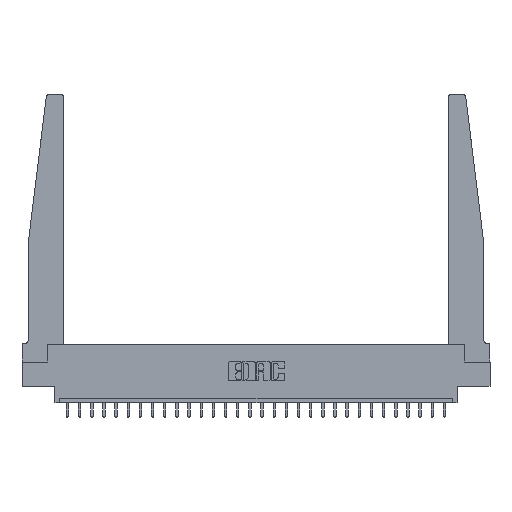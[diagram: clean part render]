
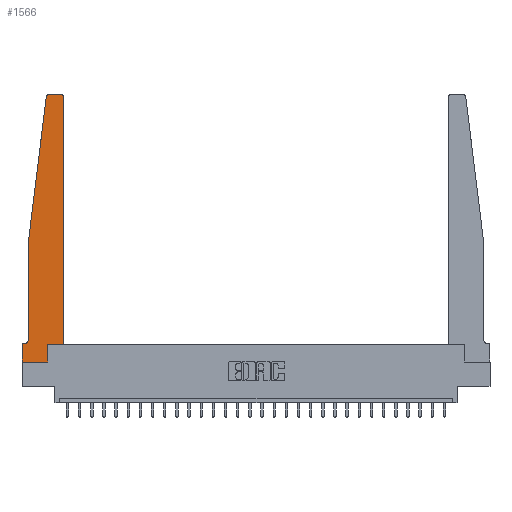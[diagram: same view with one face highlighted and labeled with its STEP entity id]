
A CAD part, top view. The second image highlights one B-rep face of the part: STEP entity #1566.
In plain terms, the highlighted planar face has unit normal (0, 0, 1).
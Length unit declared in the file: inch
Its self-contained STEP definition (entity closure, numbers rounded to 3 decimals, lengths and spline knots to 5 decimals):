
#101 = DIRECTION ( 'NONE',  ( 1., 0., 0. ) ) ;
#103 = VECTOR ( 'NONE', #4401, 39.37008 ) ;
#398 = DIRECTION ( 'NONE',  ( 1., 0., 0. ) ) ;
#920 = VERTEX_POINT ( 'NONE', #13990 ) ;
#1068 = VERTEX_POINT ( 'NONE', #12754 ) ;
#1566 = ADVANCED_FACE ( 'NONE', ( #23547 ), #2660, .T. ) ;
#1679 = DIRECTION ( 'NONE',  ( 0., 0., 1. ) ) ;
#1806 = CIRCLE ( 'NONE', #14305, 0.05 ) ;
#2044 = VECTOR ( 'NONE', #18369, 39.37008 ) ;
#2407 = ORIENTED_EDGE ( 'NONE', *, *, #11332, .T. ) ;
#2491 = VECTOR ( 'NONE', #23407, 39.37008 ) ;
#2496 = VERTEX_POINT ( 'NONE', #19792 ) ;
#2614 = EDGE_CURVE ( 'NONE', #12104, #22840, #1806, .T. ) ;
#2660 = PLANE ( 'NONE',  #24879 ) ;
#2758 = EDGE_CURVE ( 'NONE', #920, #1068, #15734, .T. ) ;
#3338 = CARTESIAN_POINT ( 'NONE',  ( 0., 0., 0.37 ) ) ;
#4401 = DIRECTION ( 'NONE',  ( 0., -1., 0. ) ) ;
#4790 = CARTESIAN_POINT ( 'NONE',  ( 0.395, 2.75, 0.37 ) ) ;
#5410 = DIRECTION ( 'NONE',  ( 0., -1., 0. ) ) ;
#5711 = EDGE_CURVE ( 'NONE', #12554, #6674, #12790, .T. ) ;
#6379 = EDGE_CURVE ( 'NONE', #22840, #8164, #20290, .T. ) ;
#6415 = CARTESIAN_POINT ( 'NONE',  ( 0.27653, 2.72, 0.37 ) ) ;
#6600 = LINE ( 'NONE', #12764, #20435 ) ;
#6674 = VERTEX_POINT ( 'NONE', #13457 ) ;
#6823 = DIRECTION ( 'NONE',  ( 0., 0., 1. ) ) ;
#6833 = ORIENTED_EDGE ( 'NONE', *, *, #6379, .T. ) ;
#6877 = CARTESIAN_POINT ( 'NONE',  ( 0.27653, 2.75, 0.37 ) ) ;
#7076 = DIRECTION ( 'NONE',  ( 0., 1., 0. ) ) ;
#7974 = CARTESIAN_POINT ( 'NONE',  ( 0., 0.1875, 0.37 ) ) ;
#8013 = DIRECTION ( 'NONE',  ( 1., 0., 0. ) ) ;
#8164 = VERTEX_POINT ( 'NONE', #7974 ) ;
#8517 = LINE ( 'NONE', #10153, #17656 ) ;
#8581 = ORIENTED_EDGE ( 'NONE', *, *, #20457, .T. ) ;
#8629 = CARTESIAN_POINT ( 'NONE',  ( 0.065, 0.2375, 0.37 ) ) ;
#8872 = CARTESIAN_POINT ( 'NONE',  ( 0.015, 0.1875, 0.37 ) ) ;
#9129 = EDGE_CURVE ( 'NONE', #6674, #13866, #22203, .T. ) ;
#9346 = LINE ( 'NONE', #3338, #16586 ) ;
#9707 = CARTESIAN_POINT ( 'NONE',  ( 0.395, 2.72, 0.37 ) ) ;
#10153 = CARTESIAN_POINT ( 'NONE',  ( 0.25, 2.75, 0.37 ) ) ;
#11116 = EDGE_CURVE ( 'NONE', #2496, #12554, #22661, .T. ) ;
#11207 = VERTEX_POINT ( 'NONE', #15752 ) ;
#11332 = EDGE_CURVE ( 'NONE', #13866, #16315, #8517, .T. ) ;
#11521 = ORIENTED_EDGE ( 'NONE', *, *, #2758, .T. ) ;
#11608 = DIRECTION ( 'NONE',  ( 0., 0., -1. ) ) ;
#11706 = ORIENTED_EDGE ( 'NONE', *, *, #23915, .T. ) ;
#12104 = VERTEX_POINT ( 'NONE', #8629 ) ;
#12554 = VERTEX_POINT ( 'NONE', #21813 ) ;
#12754 = CARTESIAN_POINT ( 'NONE',  ( 0.065, 1.25, 0.37 ) ) ;
#12764 = CARTESIAN_POINT ( 'NONE',  ( 0., 0., 0.37 ) ) ;
#12790 = LINE ( 'NONE', #18278, #2044 ) ;
#12798 = EDGE_CURVE ( 'NONE', #16315, #920, #21015, .T. ) ;
#13457 = CARTESIAN_POINT ( 'NONE',  ( 0.425, 2.72, 0.37 ) ) ;
#13866 = VERTEX_POINT ( 'NONE', #4790 ) ;
#13990 = CARTESIAN_POINT ( 'NONE',  ( 0.24675, 2.72367, 0.37 ) ) ;
#14097 = EDGE_LOOP ( 'NONE', ( #2407, #24388, #11521, #17428, #21417, #6833, #22710, #11706, #8581, #17338, #22686, #16349 ) ) ;
#14305 = AXIS2_PLACEMENT_3D ( 'NONE', #23633, #11608, #17682 ) ;
#14553 = EDGE_CURVE ( 'NONE', #1068, #12104, #23428, .T. ) ;
#14557 = LINE ( 'NONE', #18608, #23951 ) ;
#14716 = CARTESIAN_POINT ( 'NONE',  ( 0.065, 1.25, 0.37 ) ) ;
#14843 = VECTOR ( 'NONE', #101, 39.37008 ) ;
#14853 = CARTESIAN_POINT ( 'NONE',  ( 0., 0., 0.37 ) ) ;
#15599 = AXIS2_PLACEMENT_3D ( 'NONE', #6415, #20471, #398 ) ;
#15734 = LINE ( 'NONE', #17209, #2491 ) ;
#15752 = CARTESIAN_POINT ( 'NONE',  ( 0.2605, 0., 0.37 ) ) ;
#16221 = VECTOR ( 'NONE', #17805, 39.37008 ) ;
#16315 = VERTEX_POINT ( 'NONE', #6877 ) ;
#16349 = ORIENTED_EDGE ( 'NONE', *, *, #9129, .T. ) ;
#16586 = VECTOR ( 'NONE', #5410, 39.37008 ) ;
#17209 = CARTESIAN_POINT ( 'NONE',  ( 0.065, 1.25, 0.37 ) ) ;
#17338 = ORIENTED_EDGE ( 'NONE', *, *, #11116, .T. ) ;
#17428 = ORIENTED_EDGE ( 'NONE', *, *, #14553, .T. ) ;
#17656 = VECTOR ( 'NONE', #18333, 39.37008 ) ;
#17682 = DIRECTION ( 'NONE',  ( -1., 0., 0. ) ) ;
#17704 = EDGE_CURVE ( 'NONE', #8164, #25047, #9346, .T. ) ;
#17805 = DIRECTION ( 'NONE',  ( -1., 0., 0. ) ) ;
#18278 = CARTESIAN_POINT ( 'NONE',  ( 0.425, 0.18, 0.37 ) ) ;
#18333 = DIRECTION ( 'NONE',  ( -1., 0., 0. ) ) ;
#18369 = DIRECTION ( 'NONE',  ( 0., 1., 0. ) ) ;
#18608 = CARTESIAN_POINT ( 'NONE',  ( 0.2605, 0.18, 0.37 ) ) ;
#18828 = DIRECTION ( 'NONE',  ( 1., 0., 0. ) ) ;
#19792 = CARTESIAN_POINT ( 'NONE',  ( 0.2605, 0.18, 0.37 ) ) ;
#20290 = LINE ( 'NONE', #21423, #16221 ) ;
#20435 = VECTOR ( 'NONE', #18828, 39.37008 ) ;
#20457 = EDGE_CURVE ( 'NONE', #11207, #2496, #14557, .T. ) ;
#20471 = DIRECTION ( 'NONE',  ( 0., 0., 1. ) ) ;
#21015 = CIRCLE ( 'NONE', #15599, 0.03 ) ;
#21417 = ORIENTED_EDGE ( 'NONE', *, *, #2614, .T. ) ;
#21423 = CARTESIAN_POINT ( 'NONE',  ( 0.065, 0.1875, 0.37 ) ) ;
#21813 = CARTESIAN_POINT ( 'NONE',  ( 0.425, 0.18, 0.37 ) ) ;
#21849 = CARTESIAN_POINT ( 'NONE',  ( 0.425, 0.18, 0.37 ) ) ;
#21919 = AXIS2_PLACEMENT_3D ( 'NONE', #9707, #1679, #8013 ) ;
#22203 = CIRCLE ( 'NONE', #21919, 0.03 ) ;
#22661 = LINE ( 'NONE', #21849, #14843 ) ;
#22686 = ORIENTED_EDGE ( 'NONE', *, *, #5711, .T. ) ;
#22706 = CARTESIAN_POINT ( 'NONE',  ( 0., 0.1875, 0.37 ) ) ;
#22710 = ORIENTED_EDGE ( 'NONE', *, *, #17704, .T. ) ;
#22840 = VERTEX_POINT ( 'NONE', #8872 ) ;
#23407 = DIRECTION ( 'NONE',  ( -0.122, -0.992, 0. ) ) ;
#23428 = LINE ( 'NONE', #14716, #103 ) ;
#23547 = FACE_OUTER_BOUND ( 'NONE', #14097, .T. ) ;
#23633 = CARTESIAN_POINT ( 'NONE',  ( 0.015, 0.2375, 0.37 ) ) ;
#23915 = EDGE_CURVE ( 'NONE', #25047, #11207, #6600, .T. ) ;
#23951 = VECTOR ( 'NONE', #7076, 39.37008 ) ;
#24388 = ORIENTED_EDGE ( 'NONE', *, *, #12798, .T. ) ;
#24879 = AXIS2_PLACEMENT_3D ( 'NONE', #22706, #6823, #24917 ) ;
#24917 = DIRECTION ( 'NONE',  ( 1., 0., 0. ) ) ;
#25047 = VERTEX_POINT ( 'NONE', #14853 ) ;
